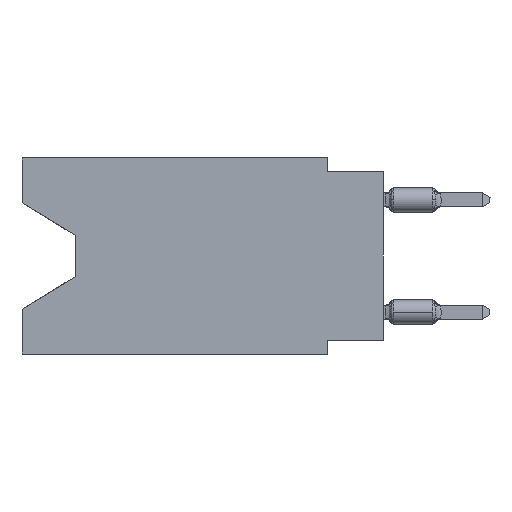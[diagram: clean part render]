
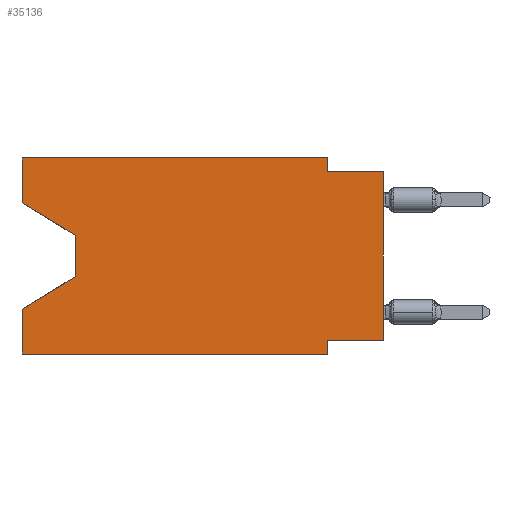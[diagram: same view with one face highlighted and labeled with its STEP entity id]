
A CAD part, left-side view. The second image highlights one B-rep face of the part: STEP entity #35136.
In plain terms, the highlighted planar face has unit normal (-1, 0, 0).
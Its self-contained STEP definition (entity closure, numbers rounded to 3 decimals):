
#1912 = EDGE_CURVE ( 'NONE', #40205, #20336, #12222, .T. ) ;
#2075 = EDGE_CURVE ( 'NONE', #40205, #5839, #13874, .T. ) ;
#2995 = ORIENTED_EDGE ( 'NONE', *, *, #7274, .F. ) ;
#3014 = VERTEX_POINT ( 'NONE', #8715 ) ;
#3054 = EDGE_CURVE ( 'NONE', #11784, #20221, #33966, .T. ) ;
#3457 = CARTESIAN_POINT ( 'NONE',  ( 0., 2.54, -8.89 ) ) ;
#4172 = CARTESIAN_POINT ( 'NONE',  ( 0., 2.54, -8.89 ) ) ;
#4512 = DIRECTION ( 'NONE',  ( 0., -1., 0. ) ) ;
#5106 = CARTESIAN_POINT ( 'NONE',  ( 0., 2.54, 0. ) ) ;
#5574 = EDGE_CURVE ( 'NONE', #32932, #7583, #39555, .T. ) ;
#5723 = DIRECTION ( 'NONE',  ( 0., 0., -1. ) ) ;
#5757 = CARTESIAN_POINT ( 'NONE',  ( 0., 2.54, 0. ) ) ;
#5807 = VECTOR ( 'NONE', #33501, 1000. ) ;
#5839 = VERTEX_POINT ( 'NONE', #46238 ) ;
#6326 = ORIENTED_EDGE ( 'NONE', *, *, #10012, .F. ) ;
#6646 = CARTESIAN_POINT ( 'NONE',  ( 0., 0., 0. ) ) ;
#6895 = ORIENTED_EDGE ( 'NONE', *, *, #1912, .T. ) ;
#7274 = EDGE_CURVE ( 'NONE', #24379, #11784, #15800, .T. ) ;
#7583 = VERTEX_POINT ( 'NONE', #33022 ) ;
#8441 = LINE ( 'NONE', #38024, #9280 ) ;
#8500 = ORIENTED_EDGE ( 'NONE', *, *, #15265, .T. ) ;
#8715 = CARTESIAN_POINT ( 'NONE',  ( 0., 0., -8.255 ) ) ;
#9258 = CARTESIAN_POINT ( 'NONE',  ( 0., 16.383, -8.89 ) ) ;
#9280 = VECTOR ( 'NONE', #45722, 1000. ) ;
#9307 = EDGE_CURVE ( 'NONE', #34970, #24379, #26293, .T. ) ;
#10012 = EDGE_CURVE ( 'NONE', #20221, #44360, #40536, .T. ) ;
#10277 = DIRECTION ( 'NONE',  ( 0., 1., 0. ) ) ;
#10334 = CARTESIAN_POINT ( 'NONE',  ( 0., 16.383, -2.038 ) ) ;
#11784 = VERTEX_POINT ( 'NONE', #5757 ) ;
#12109 = ORIENTED_EDGE ( 'NONE', *, *, #47527, .T. ) ;
#12222 = LINE ( 'NONE', #30740, #21842 ) ;
#12570 = VECTOR ( 'NONE', #24914, 1000. ) ;
#12778 = EDGE_CURVE ( 'NONE', #14254, #20336, #41637, .T. ) ;
#12985 = DIRECTION ( 'NONE',  ( 0., 0., 1. ) ) ;
#13874 = LINE ( 'NONE', #14116, #27211 ) ;
#14116 = CARTESIAN_POINT ( 'NONE',  ( 0., 16.383, 0. ) ) ;
#14208 = ORIENTED_EDGE ( 'NONE', *, *, #5574, .T. ) ;
#14254 = VERTEX_POINT ( 'NONE', #34853 ) ;
#14697 = FACE_OUTER_BOUND ( 'NONE', #36162, .T. ) ;
#15265 = EDGE_CURVE ( 'NONE', #7583, #5839, #8441, .T. ) ;
#15800 = LINE ( 'NONE', #34315, #36678 ) ;
#16881 = ORIENTED_EDGE ( 'NONE', *, *, #2075, .F. ) ;
#17516 = DIRECTION ( 'NONE',  ( 0., -0.855, -0.519 ) ) ;
#17915 = LINE ( 'NONE', #6646, #12570 ) ;
#18642 = CARTESIAN_POINT ( 'NONE',  ( 0., 0., -0.635 ) ) ;
#19475 = VECTOR ( 'NONE', #17516, 1000. ) ;
#19653 = DIRECTION ( 'NONE',  ( 0., -1., 0. ) ) ;
#20221 = VERTEX_POINT ( 'NONE', #24622 ) ;
#20336 = VERTEX_POINT ( 'NONE', #3457 ) ;
#20445 = VECTOR ( 'NONE', #33507, 1000. ) ;
#21460 = CARTESIAN_POINT ( 'NONE',  ( 0., 16.383, 0. ) ) ;
#21842 = VECTOR ( 'NONE', #19653, 1000. ) ;
#23287 = ORIENTED_EDGE ( 'NONE', *, *, #40638, .T. ) ;
#24117 = CARTESIAN_POINT ( 'NONE',  ( 0., 0., -0.635 ) ) ;
#24379 = VERTEX_POINT ( 'NONE', #21460 ) ;
#24622 = CARTESIAN_POINT ( 'NONE',  ( 0., 2.54, -0.635 ) ) ;
#24914 = DIRECTION ( 'NONE',  ( 0., 0., 1. ) ) ;
#26293 = LINE ( 'NONE', #30791, #42208 ) ;
#27211 = VECTOR ( 'NONE', #39607, 1000. ) ;
#27650 = LINE ( 'NONE', #10334, #19475 ) ;
#28261 = CARTESIAN_POINT ( 'NONE',  ( 0., 13.97, -3.505 ) ) ;
#29199 = AXIS2_PLACEMENT_3D ( 'NONE', #44284, #31215, #5723 ) ;
#29706 = VECTOR ( 'NONE', #10277, 1000. ) ;
#30740 = CARTESIAN_POINT ( 'NONE',  ( 0., 16.383, -8.89 ) ) ;
#30791 = CARTESIAN_POINT ( 'NONE',  ( 0., 16.383, 0. ) ) ;
#31215 = DIRECTION ( 'NONE',  ( 1., 0., 0. ) ) ;
#31443 = CARTESIAN_POINT ( 'NONE',  ( 0., 0., -8.255 ) ) ;
#31809 = CARTESIAN_POINT ( 'NONE',  ( 0., 16.383, -2.038 ) ) ;
#32212 = EDGE_CURVE ( 'NONE', #3014, #14254, #35767, .T. ) ;
#32932 = VERTEX_POINT ( 'NONE', #38245 ) ;
#33022 = CARTESIAN_POINT ( 'NONE',  ( 0., 13.97, -5.385 ) ) ;
#33345 = DIRECTION ( 'NONE',  ( 0., -1., 0. ) ) ;
#33501 = DIRECTION ( 'NONE',  ( 0., 0., -1. ) ) ;
#33507 = DIRECTION ( 'NONE',  ( 0., 0., -1. ) ) ;
#33966 = LINE ( 'NONE', #5106, #20445 ) ;
#34315 = CARTESIAN_POINT ( 'NONE',  ( 0., 16.383, 0. ) ) ;
#34853 = CARTESIAN_POINT ( 'NONE',  ( 0., 2.54, -8.255 ) ) ;
#34970 = VERTEX_POINT ( 'NONE', #31809 ) ;
#35136 = ADVANCED_FACE ( 'NONE', ( #14697 ), #36829, .F. ) ;
#35642 = ORIENTED_EDGE ( 'NONE', *, *, #3054, .F. ) ;
#35767 = LINE ( 'NONE', #31443, #29706 ) ;
#36162 = EDGE_LOOP ( 'NONE', ( #23287, #14208, #8500, #16881, #6895, #40197, #38348, #12109, #6326, #35642, #2995, #43748 ) ) ;
#36678 = VECTOR ( 'NONE', #4512, 1000. ) ;
#36829 = PLANE ( 'NONE',  #29199 ) ;
#38024 = CARTESIAN_POINT ( 'NONE',  ( 0., 13.97, -5.385 ) ) ;
#38245 = CARTESIAN_POINT ( 'NONE',  ( 0., 13.97, -3.505 ) ) ;
#38348 = ORIENTED_EDGE ( 'NONE', *, *, #32212, .F. ) ;
#39555 = LINE ( 'NONE', #28261, #43018 ) ;
#39607 = DIRECTION ( 'NONE',  ( 0., 0., 1. ) ) ;
#40197 = ORIENTED_EDGE ( 'NONE', *, *, #12778, .F. ) ;
#40205 = VERTEX_POINT ( 'NONE', #9258 ) ;
#40250 = DIRECTION ( 'NONE',  ( 0., 0., -1. ) ) ;
#40536 = LINE ( 'NONE', #18642, #42270 ) ;
#40638 = EDGE_CURVE ( 'NONE', #34970, #32932, #27650, .T. ) ;
#41637 = LINE ( 'NONE', #4172, #5807 ) ;
#42208 = VECTOR ( 'NONE', #12985, 1000. ) ;
#42270 = VECTOR ( 'NONE', #33345, 1000. ) ;
#43018 = VECTOR ( 'NONE', #40250, 1000. ) ;
#43748 = ORIENTED_EDGE ( 'NONE', *, *, #9307, .F. ) ;
#44284 = CARTESIAN_POINT ( 'NONE',  ( 0., 16.383, 0. ) ) ;
#44360 = VERTEX_POINT ( 'NONE', #24117 ) ;
#45722 = DIRECTION ( 'NONE',  ( 0., 0.855, -0.519 ) ) ;
#46238 = CARTESIAN_POINT ( 'NONE',  ( 0., 16.383, -6.852 ) ) ;
#47527 = EDGE_CURVE ( 'NONE', #3014, #44360, #17915, .T. ) ;
